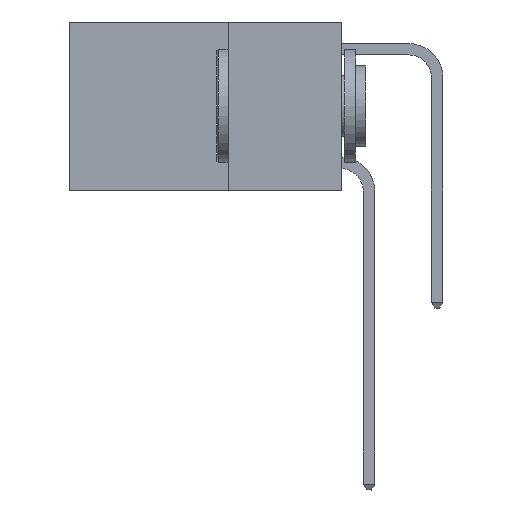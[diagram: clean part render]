
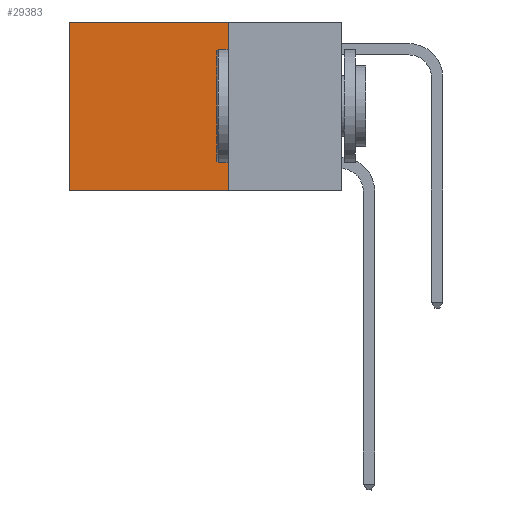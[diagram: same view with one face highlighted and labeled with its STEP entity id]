
A CAD part, left-side view. The second image highlights one B-rep face of the part: STEP entity #29383.
In plain terms, the highlighted planar face has unit normal (-1, 0, 0).
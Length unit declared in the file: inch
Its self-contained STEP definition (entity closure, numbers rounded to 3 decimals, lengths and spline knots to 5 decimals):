
#433 = VECTOR ( 'NONE', #14147, 39.37008 ) ;
#2933 = VECTOR ( 'NONE', #25438, 39.37008 ) ;
#5735 = FACE_OUTER_BOUND ( 'NONE', #13721, .T. ) ;
#5794 = CARTESIAN_POINT ( 'NONE',  ( 0.2625, 0.6, 0. ) ) ;
#7362 = ORIENTED_EDGE ( 'NONE', *, *, #12286, .F. ) ;
#7487 = CARTESIAN_POINT ( 'NONE',  ( 0.2625, 0.6, 0. ) ) ;
#7646 = PLANE ( 'NONE',  #22161 ) ;
#8552 = CARTESIAN_POINT ( 'NONE',  ( 0.2625, 0.25, -0.37 ) ) ;
#9157 = VECTOR ( 'NONE', #25484, 39.37008 ) ;
#9881 = LINE ( 'NONE', #7487, #433 ) ;
#10000 = VERTEX_POINT ( 'NONE', #8552 ) ;
#10788 = LINE ( 'NONE', #20438, #22857 ) ;
#12286 = EDGE_CURVE ( 'NONE', #20198, #10000, #25794, .T. ) ;
#13237 = CARTESIAN_POINT ( 'NONE',  ( 0.2625, 0.6, -0.37 ) ) ;
#13277 = EDGE_CURVE ( 'NONE', #20198, #26215, #10788, .T. ) ;
#13721 = EDGE_LOOP ( 'NONE', ( #27593, #19468, #7362, #31053 ) ) ;
#14013 = LINE ( 'NONE', #20834, #2933 ) ;
#14147 = DIRECTION ( 'NONE',  ( 0., 0., -1. ) ) ;
#14920 = DIRECTION ( 'NONE',  ( 1., 0., 0. ) ) ;
#15839 = CARTESIAN_POINT ( 'NONE',  ( 0.2625, 0.25, 0. ) ) ;
#17288 = CARTESIAN_POINT ( 'NONE',  ( 0.2625, 0.25, 0. ) ) ;
#17768 = VERTEX_POINT ( 'NONE', #13237 ) ;
#19468 = ORIENTED_EDGE ( 'NONE', *, *, #27140, .F. ) ;
#20198 = VERTEX_POINT ( 'NONE', #27859 ) ;
#20438 = CARTESIAN_POINT ( 'NONE',  ( 0.2625, 0.25, 0. ) ) ;
#20834 = CARTESIAN_POINT ( 'NONE',  ( 0.2625, 0.25, -0.37 ) ) ;
#22161 = AXIS2_PLACEMENT_3D ( 'NONE', #17288, #14920, #24576 ) ;
#22215 = EDGE_CURVE ( 'NONE', #26215, #17768, #9881, .T. ) ;
#22857 = VECTOR ( 'NONE', #30138, 39.37008 ) ;
#24576 = DIRECTION ( 'NONE',  ( 0., 0., -1. ) ) ;
#25438 = DIRECTION ( 'NONE',  ( 0., 1., 0. ) ) ;
#25484 = DIRECTION ( 'NONE',  ( 0., 0., -1. ) ) ;
#25794 = LINE ( 'NONE', #15839, #9157 ) ;
#26215 = VERTEX_POINT ( 'NONE', #5794 ) ;
#27140 = EDGE_CURVE ( 'NONE', #10000, #17768, #14013, .T. ) ;
#27593 = ORIENTED_EDGE ( 'NONE', *, *, #22215, .T. ) ;
#27859 = CARTESIAN_POINT ( 'NONE',  ( 0.2625, 0.25, 0. ) ) ;
#29383 = ADVANCED_FACE ( 'NONE', ( #5735 ), #7646, .F. ) ;
#30138 = DIRECTION ( 'NONE',  ( 0., 1., 0. ) ) ;
#31053 = ORIENTED_EDGE ( 'NONE', *, *, #13277, .T. ) ;
